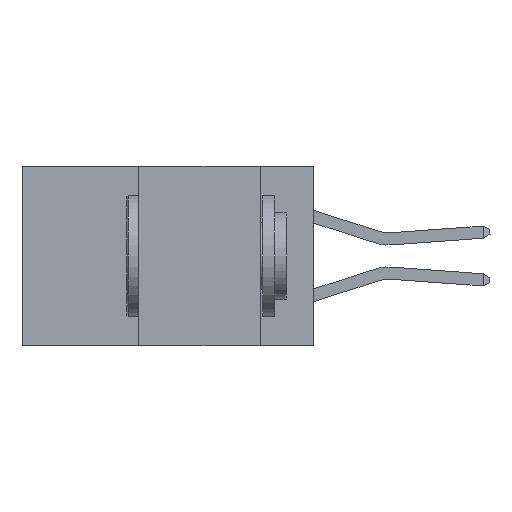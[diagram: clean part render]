
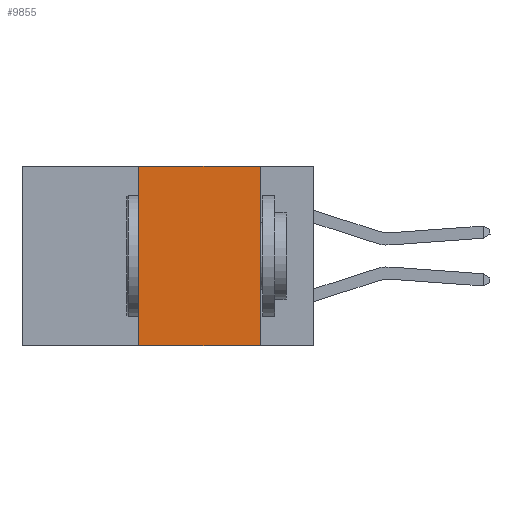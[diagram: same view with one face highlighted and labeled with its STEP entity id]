
A CAD part, left-side view. The second image highlights one B-rep face of the part: STEP entity #9855.
In plain terms, the highlighted planar face has unit normal (-1, 0, 0).
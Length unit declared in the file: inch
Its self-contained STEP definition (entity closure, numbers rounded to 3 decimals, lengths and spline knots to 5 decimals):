
#40 = ORIENTED_EDGE ( 'NONE', *, *, #269, .F. ) ;
#269 = EDGE_CURVE ( 'NONE', #1232, #6285, #17205, .T. ) ;
#341 = DIRECTION ( 'NONE',  ( 0., -1., 0. ) ) ;
#442 = CARTESIAN_POINT ( 'NONE',  ( 0., 0.11, -0.37 ) ) ;
#897 = LINE ( 'NONE', #10566, #10272 ) ;
#1232 = VERTEX_POINT ( 'NONE', #3567 ) ;
#2621 = VECTOR ( 'NONE', #7483, 39.37008 ) ;
#3436 = LINE ( 'NONE', #20321, #7852 ) ;
#3498 = VERTEX_POINT ( 'NONE', #7244 ) ;
#3567 = CARTESIAN_POINT ( 'NONE',  ( 0., 0.36, -0.37 ) ) ;
#3755 = CARTESIAN_POINT ( 'NONE',  ( 0., 0.6, 0. ) ) ;
#4402 = ORIENTED_EDGE ( 'NONE', *, *, #16300, .F. ) ;
#5660 = DIRECTION ( 'NONE',  ( 1., 0., 0. ) ) ;
#6285 = VERTEX_POINT ( 'NONE', #12850 ) ;
#7244 = CARTESIAN_POINT ( 'NONE',  ( 0., 0.11, 0. ) ) ;
#7483 = DIRECTION ( 'NONE',  ( 0., 0., 1. ) ) ;
#7632 = FACE_OUTER_BOUND ( 'NONE', #22809, .T. ) ;
#7852 = VECTOR ( 'NONE', #341, 39.37008 ) ;
#7878 = VERTEX_POINT ( 'NONE', #442 ) ;
#8620 = DIRECTION ( 'NONE',  ( 0., 0., -1. ) ) ;
#9232 = CARTESIAN_POINT ( 'NONE',  ( 0., 0.36, 0. ) ) ;
#9855 = ADVANCED_FACE ( 'NONE', ( #7632 ), #18250, .F. ) ;
#10003 = ORIENTED_EDGE ( 'NONE', *, *, #22599, .T. ) ;
#10272 = VECTOR ( 'NONE', #8620, 39.37008 ) ;
#10566 = CARTESIAN_POINT ( 'NONE',  ( 0., 0.11, 0. ) ) ;
#10664 = VECTOR ( 'NONE', #21481, 39.37008 ) ;
#12850 = CARTESIAN_POINT ( 'NONE',  ( 0., 0.36, 0. ) ) ;
#14245 = ORIENTED_EDGE ( 'NONE', *, *, #18554, .F. ) ;
#15836 = AXIS2_PLACEMENT_3D ( 'NONE', #3755, #5660, #18327 ) ;
#15995 = LINE ( 'NONE', #17874, #10664 ) ;
#16300 = EDGE_CURVE ( 'NONE', #3498, #7878, #897, .T. ) ;
#17205 = LINE ( 'NONE', #9232, #2621 ) ;
#17874 = CARTESIAN_POINT ( 'NONE',  ( 0., 0.6, 0. ) ) ;
#18250 = PLANE ( 'NONE',  #15836 ) ;
#18327 = DIRECTION ( 'NONE',  ( 0., 0., -1. ) ) ;
#18554 = EDGE_CURVE ( 'NONE', #6285, #3498, #15995, .T. ) ;
#20321 = CARTESIAN_POINT ( 'NONE',  ( 0., 0.6, -0.37 ) ) ;
#21481 = DIRECTION ( 'NONE',  ( 0., -1., 0. ) ) ;
#22599 = EDGE_CURVE ( 'NONE', #1232, #7878, #3436, .T. ) ;
#22809 = EDGE_LOOP ( 'NONE', ( #4402, #14245, #40, #10003 ) ) ;
